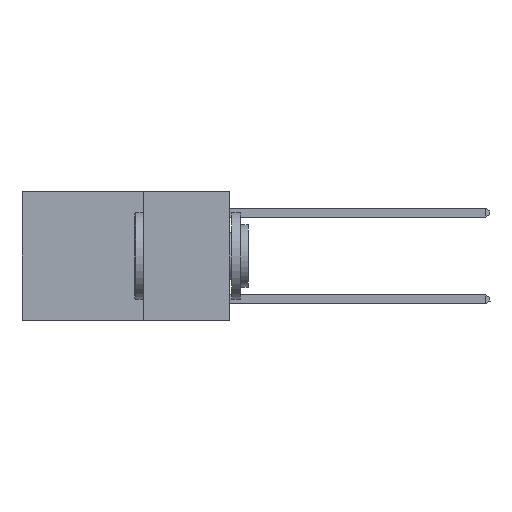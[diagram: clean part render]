
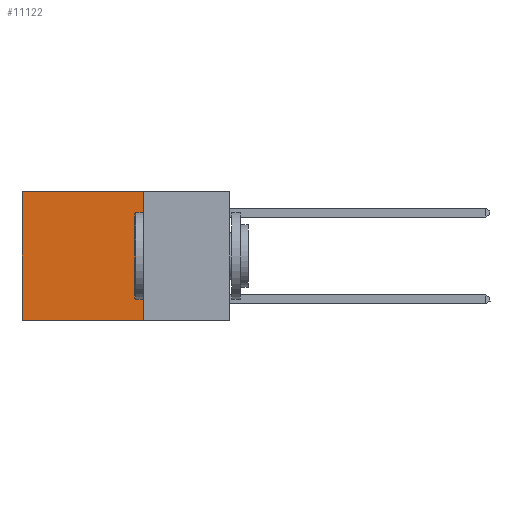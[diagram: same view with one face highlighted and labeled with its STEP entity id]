
A CAD part, left-side view. The second image highlights one B-rep face of the part: STEP entity #11122.
In plain terms, the highlighted planar face has unit normal (-1, 0, 0).
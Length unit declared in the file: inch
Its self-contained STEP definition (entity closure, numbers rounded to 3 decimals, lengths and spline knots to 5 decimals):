
#340 = DIRECTION ( 'NONE',  ( 0., 1., 0. ) ) ;
#541 = DIRECTION ( 'NONE',  ( 0., 0., -1. ) ) ;
#1703 = VERTEX_POINT ( 'NONE', #10582 ) ;
#1792 = VERTEX_POINT ( 'NONE', #11797 ) ;
#1883 = LINE ( 'NONE', #5633, #8893 ) ;
#1894 = PLANE ( 'NONE',  #6913 ) ;
#2525 = CARTESIAN_POINT ( 'NONE',  ( 0.2625, 0.25, 0. ) ) ;
#2689 = DIRECTION ( 'NONE',  ( 0., 0., -1. ) ) ;
#2781 = LINE ( 'NONE', #6290, #4642 ) ;
#3010 = EDGE_CURVE ( 'NONE', #1703, #10717, #4323, .T. ) ;
#3463 = EDGE_CURVE ( 'NONE', #10717, #1792, #1883, .T. ) ;
#4199 = ORIENTED_EDGE ( 'NONE', *, *, #3010, .F. ) ;
#4323 = LINE ( 'NONE', #2525, #5852 ) ;
#4642 = VECTOR ( 'NONE', #541, 39.37008 ) ;
#4868 = LINE ( 'NONE', #10907, #6849 ) ;
#5503 = CARTESIAN_POINT ( 'NONE',  ( 0.2625, 0.25, -0.37 ) ) ;
#5633 = CARTESIAN_POINT ( 'NONE',  ( 0.2625, 0.25, -0.37 ) ) ;
#5852 = VECTOR ( 'NONE', #11321, 39.37008 ) ;
#6055 = CARTESIAN_POINT ( 'NONE',  ( 0.2625, 0.6, 0. ) ) ;
#6210 = ORIENTED_EDGE ( 'NONE', *, *, #11441, .T. ) ;
#6290 = CARTESIAN_POINT ( 'NONE',  ( 0.2625, 0.6, 0. ) ) ;
#6666 = CARTESIAN_POINT ( 'NONE',  ( 0.2625, 0.25, 0. ) ) ;
#6723 = ORIENTED_EDGE ( 'NONE', *, *, #3463, .F. ) ;
#6849 = VECTOR ( 'NONE', #340, 39.37008 ) ;
#6913 = AXIS2_PLACEMENT_3D ( 'NONE', #6666, #8550, #2689 ) ;
#7096 = ORIENTED_EDGE ( 'NONE', *, *, #8976, .T. ) ;
#8550 = DIRECTION ( 'NONE',  ( 1., 0., 0. ) ) ;
#8630 = FACE_OUTER_BOUND ( 'NONE', #10587, .T. ) ;
#8893 = VECTOR ( 'NONE', #9514, 39.37008 ) ;
#8976 = EDGE_CURVE ( 'NONE', #1703, #10133, #4868, .T. ) ;
#9514 = DIRECTION ( 'NONE',  ( 0., 1., 0. ) ) ;
#10133 = VERTEX_POINT ( 'NONE', #6055 ) ;
#10582 = CARTESIAN_POINT ( 'NONE',  ( 0.2625, 0.25, 0. ) ) ;
#10587 = EDGE_LOOP ( 'NONE', ( #6210, #6723, #4199, #7096 ) ) ;
#10717 = VERTEX_POINT ( 'NONE', #5503 ) ;
#10907 = CARTESIAN_POINT ( 'NONE',  ( 0.2625, 0.25, 0. ) ) ;
#11122 = ADVANCED_FACE ( 'NONE', ( #8630 ), #1894, .F. ) ;
#11321 = DIRECTION ( 'NONE',  ( 0., 0., -1. ) ) ;
#11441 = EDGE_CURVE ( 'NONE', #10133, #1792, #2781, .T. ) ;
#11797 = CARTESIAN_POINT ( 'NONE',  ( 0.2625, 0.6, -0.37 ) ) ;
